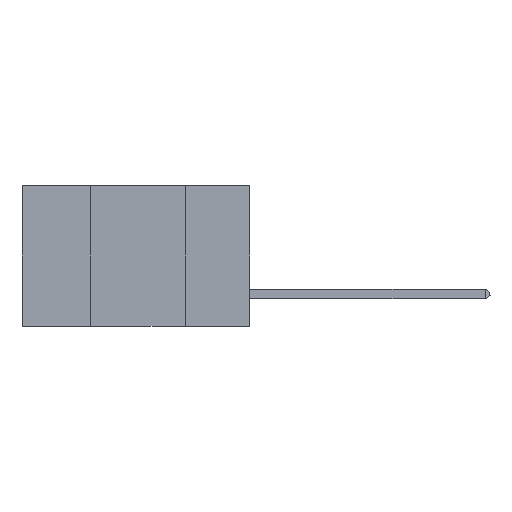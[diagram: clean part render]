
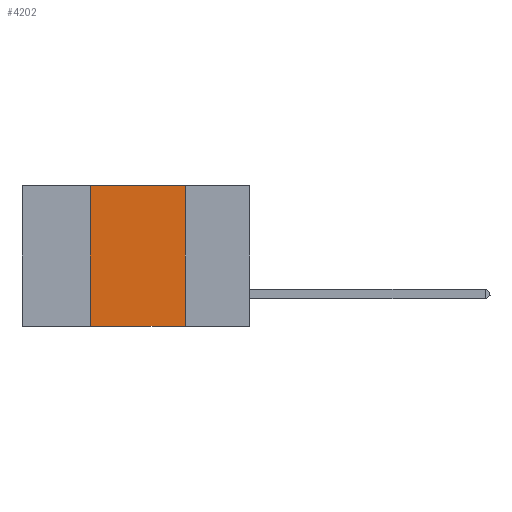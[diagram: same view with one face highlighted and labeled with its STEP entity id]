
A CAD part, left-side view. The second image highlights one B-rep face of the part: STEP entity #4202.
In plain terms, the highlighted planar face has unit normal (-1, 0, 0).
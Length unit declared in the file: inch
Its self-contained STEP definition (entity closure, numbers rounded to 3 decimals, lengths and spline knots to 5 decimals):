
#428 = CARTESIAN_POINT ( 'NONE',  ( 0., 0.42, -0.37 ) ) ;
#716 = DIRECTION ( 'NONE',  ( 0., 0., -1. ) ) ;
#983 = ORIENTED_EDGE ( 'NONE', *, *, #5905, .F. ) ;
#1663 = DIRECTION ( 'NONE',  ( 0., -1., 0. ) ) ;
#1717 = CARTESIAN_POINT ( 'NONE',  ( 0., 0.6, 0. ) ) ;
#1727 = EDGE_CURVE ( 'NONE', #10606, #4207, #7810, .T. ) ;
#1754 = CARTESIAN_POINT ( 'NONE',  ( 0., 0.42, 0. ) ) ;
#3226 = CARTESIAN_POINT ( 'NONE',  ( 0., 0.42, 0. ) ) ;
#4110 = VECTOR ( 'NONE', #4288, 39.37008 ) ;
#4202 = ADVANCED_FACE ( 'NONE', ( #4732 ), #4587, .F. ) ;
#4207 = VERTEX_POINT ( 'NONE', #1754 ) ;
#4288 = DIRECTION ( 'NONE',  ( 0., 0., -1. ) ) ;
#4587 = PLANE ( 'NONE',  #4922 ) ;
#4732 = FACE_OUTER_BOUND ( 'NONE', #8939, .T. ) ;
#4922 = AXIS2_PLACEMENT_3D ( 'NONE', #1717, #6494, #716 ) ;
#5653 = VERTEX_POINT ( 'NONE', #9344 ) ;
#5905 = EDGE_CURVE ( 'NONE', #4207, #5653, #10634, .T. ) ;
#6188 = VECTOR ( 'NONE', #1663, 39.37008 ) ;
#6283 = VECTOR ( 'NONE', #11072, 39.37008 ) ;
#6393 = EDGE_CURVE ( 'NONE', #5653, #10887, #9578, .T. ) ;
#6494 = DIRECTION ( 'NONE',  ( 1., 0., 0. ) ) ;
#6618 = CARTESIAN_POINT ( 'NONE',  ( 0., 0.17, -0.37 ) ) ;
#7043 = EDGE_CURVE ( 'NONE', #10606, #10887, #10761, .T. ) ;
#7427 = ORIENTED_EDGE ( 'NONE', *, *, #1727, .F. ) ;
#7810 = LINE ( 'NONE', #3226, #6283 ) ;
#8160 = VECTOR ( 'NONE', #9192, 39.37008 ) ;
#8388 = ORIENTED_EDGE ( 'NONE', *, *, #7043, .T. ) ;
#8939 = EDGE_LOOP ( 'NONE', ( #11470, #983, #7427, #8388 ) ) ;
#9192 = DIRECTION ( 'NONE',  ( 0., -1., 0. ) ) ;
#9344 = CARTESIAN_POINT ( 'NONE',  ( 0., 0.17, 0. ) ) ;
#9578 = LINE ( 'NONE', #10290, #4110 ) ;
#10290 = CARTESIAN_POINT ( 'NONE',  ( 0., 0.17, 0. ) ) ;
#10606 = VERTEX_POINT ( 'NONE', #428 ) ;
#10634 = LINE ( 'NONE', #11266, #6188 ) ;
#10761 = LINE ( 'NONE', #11908, #8160 ) ;
#10887 = VERTEX_POINT ( 'NONE', #6618 ) ;
#11072 = DIRECTION ( 'NONE',  ( 0., 0., 1. ) ) ;
#11266 = CARTESIAN_POINT ( 'NONE',  ( 0., 0.6, 0. ) ) ;
#11470 = ORIENTED_EDGE ( 'NONE', *, *, #6393, .F. ) ;
#11908 = CARTESIAN_POINT ( 'NONE',  ( 0., 0.6, -0.37 ) ) ;
